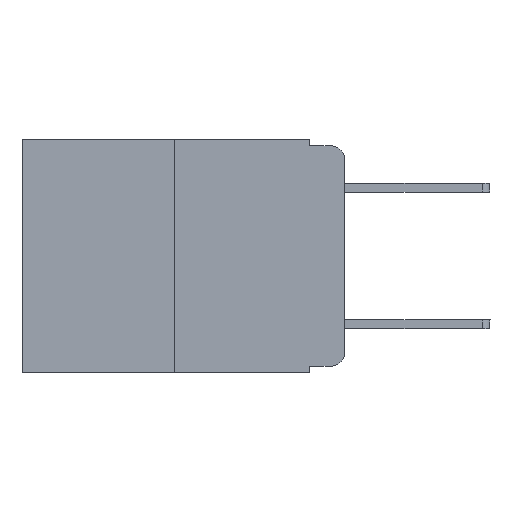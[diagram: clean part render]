
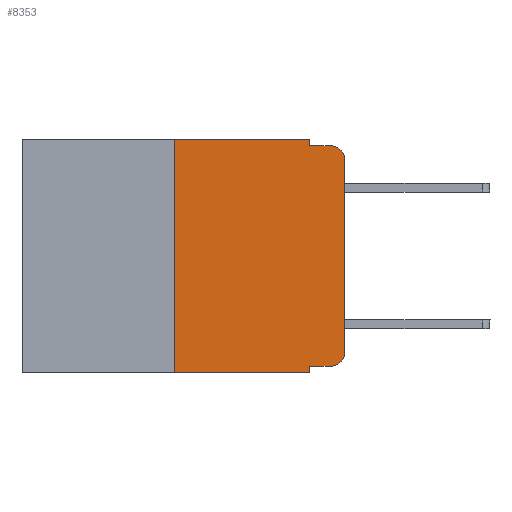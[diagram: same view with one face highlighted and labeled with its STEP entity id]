
A CAD part, left-side view. The second image highlights one B-rep face of the part: STEP entity #8353.
In plain terms, the highlighted planar face has unit normal (-1, 0, 0).
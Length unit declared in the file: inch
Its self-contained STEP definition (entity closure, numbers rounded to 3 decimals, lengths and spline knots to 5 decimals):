
#753 = CARTESIAN_POINT ( 'NONE',  ( 0., 0.051, -0.01 ) ) ;
#905 = VECTOR ( 'NONE', #13770, 39.37008 ) ;
#1023 = EDGE_CURVE ( 'NONE', #3646, #2554, #7730, .T. ) ;
#1155 = CARTESIAN_POINT ( 'NONE',  ( 0., 0., -0.03 ) ) ;
#1394 = CARTESIAN_POINT ( 'NONE',  ( 0., 0.051, 0. ) ) ;
#1718 = CARTESIAN_POINT ( 'NONE',  ( 0., 0.473, 0. ) ) ;
#1884 = ORIENTED_EDGE ( 'NONE', *, *, #1023, .T. ) ;
#2141 = LINE ( 'NONE', #15225, #905 ) ;
#2217 = FACE_OUTER_BOUND ( 'NONE', #13195, .T. ) ;
#2317 = DIRECTION ( 'NONE',  ( 0., 0., 1. ) ) ;
#2535 = CARTESIAN_POINT ( 'NONE',  ( 0., 0.051, 0. ) ) ;
#2554 = VERTEX_POINT ( 'NONE', #9086 ) ;
#2568 = DIRECTION ( 'NONE',  ( 0., 0., -1. ) ) ;
#3015 = LINE ( 'NONE', #13193, #9600 ) ;
#3047 = DIRECTION ( 'NONE',  ( 0., -1., 0. ) ) ;
#3189 = DIRECTION ( 'NONE',  ( 0., 0., -1. ) ) ;
#3315 = ORIENTED_EDGE ( 'NONE', *, *, #6232, .F. ) ;
#3421 = AXIS2_PLACEMENT_3D ( 'NONE', #6093, #7425, #6208 ) ;
#3541 = EDGE_CURVE ( 'NONE', #4590, #12296, #13550, .T. ) ;
#3641 = CARTESIAN_POINT ( 'NONE',  ( 0., 0.02, -0.03 ) ) ;
#3646 = VERTEX_POINT ( 'NONE', #14062 ) ;
#4042 = ORIENTED_EDGE ( 'NONE', *, *, #10630, .T. ) ;
#4372 = ORIENTED_EDGE ( 'NONE', *, *, #16235, .T. ) ;
#4380 = EDGE_CURVE ( 'NONE', #9029, #11545, #7419, .T. ) ;
#4467 = LINE ( 'NONE', #5436, #10596 ) ;
#4590 = VERTEX_POINT ( 'NONE', #8640 ) ;
#4738 = AXIS2_PLACEMENT_3D ( 'NONE', #3641, #15622, #4956 ) ;
#4791 = CARTESIAN_POINT ( 'NONE',  ( 0., 0.25, 0. ) ) ;
#4956 = DIRECTION ( 'NONE',  ( 0., 0., -1. ) ) ;
#5436 = CARTESIAN_POINT ( 'NONE',  ( 0., 0.473, -0.343 ) ) ;
#5800 = LINE ( 'NONE', #15056, #8877 ) ;
#5878 = VECTOR ( 'NONE', #2317, 39.37008 ) ;
#6093 = CARTESIAN_POINT ( 'NONE',  ( 0., 0.02, -0.313 ) ) ;
#6208 = DIRECTION ( 'NONE',  ( 0., 0., -1. ) ) ;
#6232 = EDGE_CURVE ( 'NONE', #14821, #11680, #3015, .T. ) ;
#6374 = AXIS2_PLACEMENT_3D ( 'NONE', #8427, #14959, #3189 ) ;
#6723 = VERTEX_POINT ( 'NONE', #1155 ) ;
#7016 = CARTESIAN_POINT ( 'NONE',  ( 0., 0.051, -0.343 ) ) ;
#7132 = EDGE_CURVE ( 'NONE', #11680, #15867, #2141, .T. ) ;
#7419 = LINE ( 'NONE', #2535, #15835 ) ;
#7425 = DIRECTION ( 'NONE',  ( -1., 0., 0. ) ) ;
#7432 = VECTOR ( 'NONE', #16443, 39.37008 ) ;
#7730 = CIRCLE ( 'NONE', #3421, 0.02 ) ;
#8353 = ADVANCED_FACE ( 'NONE', ( #2217 ), #8478, .F. ) ;
#8385 = LINE ( 'NONE', #1718, #15156 ) ;
#8427 = CARTESIAN_POINT ( 'NONE',  ( 0., 0.473, 0. ) ) ;
#8478 = PLANE ( 'NONE',  #6374 ) ;
#8640 = CARTESIAN_POINT ( 'NONE',  ( 0., 0.25, -0.343 ) ) ;
#8877 = VECTOR ( 'NONE', #14944, 39.37008 ) ;
#8988 = DIRECTION ( 'NONE',  ( 0., 0., -1. ) ) ;
#9029 = VERTEX_POINT ( 'NONE', #9777 ) ;
#9086 = CARTESIAN_POINT ( 'NONE',  ( 0., 0., -0.313 ) ) ;
#9600 = VECTOR ( 'NONE', #2568, 39.37008 ) ;
#9777 = CARTESIAN_POINT ( 'NONE',  ( 0., 0.051, -0.333 ) ) ;
#9952 = EDGE_CURVE ( 'NONE', #2554, #6723, #12854, .T. ) ;
#10375 = ORIENTED_EDGE ( 'NONE', *, *, #4380, .F. ) ;
#10596 = VECTOR ( 'NONE', #16012, 39.37008 ) ;
#10630 = EDGE_CURVE ( 'NONE', #6723, #15867, #13035, .T. ) ;
#11545 = VERTEX_POINT ( 'NONE', #7016 ) ;
#11680 = VERTEX_POINT ( 'NONE', #753 ) ;
#11777 = ORIENTED_EDGE ( 'NONE', *, *, #13826, .F. ) ;
#12227 = EDGE_CURVE ( 'NONE', #9029, #3646, #5800, .T. ) ;
#12296 = VERTEX_POINT ( 'NONE', #4791 ) ;
#12782 = CARTESIAN_POINT ( 'NONE',  ( 0., 0.02, -0.01 ) ) ;
#12854 = LINE ( 'NONE', #15590, #5878 ) ;
#13035 = CIRCLE ( 'NONE', #4738, 0.02 ) ;
#13193 = CARTESIAN_POINT ( 'NONE',  ( 0., 0.051, 0. ) ) ;
#13195 = EDGE_LOOP ( 'NONE', ( #16704, #4042, #14336, #3315, #11777, #16768, #4372, #10375, #14273, #1884 ) ) ;
#13550 = LINE ( 'NONE', #15166, #7432 ) ;
#13770 = DIRECTION ( 'NONE',  ( 0., -1., 0. ) ) ;
#13826 = EDGE_CURVE ( 'NONE', #12296, #14821, #8385, .T. ) ;
#14062 = CARTESIAN_POINT ( 'NONE',  ( 0., 0.02, -0.333 ) ) ;
#14273 = ORIENTED_EDGE ( 'NONE', *, *, #12227, .T. ) ;
#14336 = ORIENTED_EDGE ( 'NONE', *, *, #7132, .F. ) ;
#14821 = VERTEX_POINT ( 'NONE', #1394 ) ;
#14944 = DIRECTION ( 'NONE',  ( 0., -1., 0. ) ) ;
#14959 = DIRECTION ( 'NONE',  ( 1., 0., 0. ) ) ;
#15056 = CARTESIAN_POINT ( 'NONE',  ( 0., 0.051, -0.333 ) ) ;
#15156 = VECTOR ( 'NONE', #3047, 39.37008 ) ;
#15166 = CARTESIAN_POINT ( 'NONE',  ( 0., 0.25, 0. ) ) ;
#15225 = CARTESIAN_POINT ( 'NONE',  ( 0., 0.051, -0.01 ) ) ;
#15590 = CARTESIAN_POINT ( 'NONE',  ( 0., 0., 0. ) ) ;
#15622 = DIRECTION ( 'NONE',  ( -1., 0., 0. ) ) ;
#15835 = VECTOR ( 'NONE', #8988, 39.37008 ) ;
#15867 = VERTEX_POINT ( 'NONE', #12782 ) ;
#16012 = DIRECTION ( 'NONE',  ( 0., -1., 0. ) ) ;
#16235 = EDGE_CURVE ( 'NONE', #4590, #11545, #4467, .T. ) ;
#16443 = DIRECTION ( 'NONE',  ( 0., 0., 1. ) ) ;
#16704 = ORIENTED_EDGE ( 'NONE', *, *, #9952, .T. ) ;
#16768 = ORIENTED_EDGE ( 'NONE', *, *, #3541, .F. ) ;
